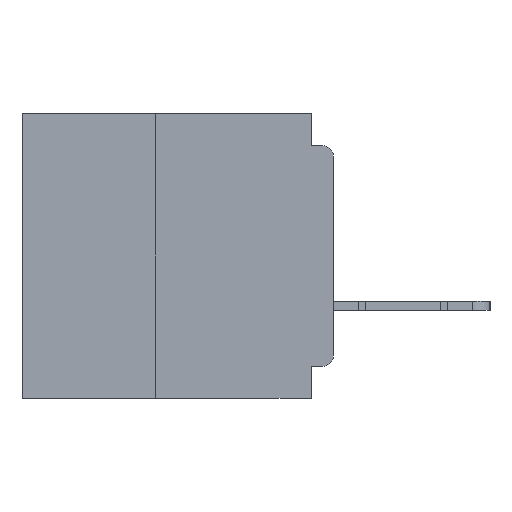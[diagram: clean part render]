
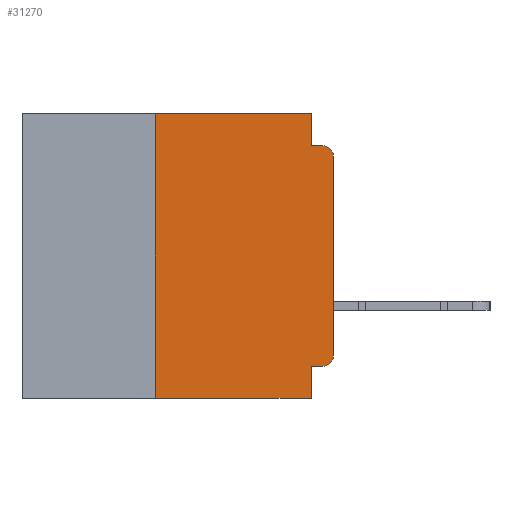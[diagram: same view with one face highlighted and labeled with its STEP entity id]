
A CAD part, left-side view. The second image highlights one B-rep face of the part: STEP entity #31270.
In plain terms, the highlighted planar face has unit normal (-1, 0, 0).
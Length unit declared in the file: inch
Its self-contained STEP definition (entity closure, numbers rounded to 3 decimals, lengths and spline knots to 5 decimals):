
#392 = EDGE_CURVE ( 'NONE', #51800, #35690, #58561, .T. ) ;
#763 = VECTOR ( 'NONE', #40756, 39.37008 ) ;
#3335 = CARTESIAN_POINT ( 'NONE',  ( 0., 0., -0.34 ) ) ;
#5136 = VERTEX_POINT ( 'NONE', #37436 ) ;
#7780 = CARTESIAN_POINT ( 'NONE',  ( 0., 0.25, -0.4 ) ) ;
#8727 = ORIENTED_EDGE ( 'NONE', *, *, #30371, .F. ) ;
#9059 = VERTEX_POINT ( 'NONE', #26474 ) ;
#10209 = DIRECTION ( 'NONE',  ( -1., 0., 0. ) ) ;
#10276 = LINE ( 'NONE', #24117, #22077 ) ;
#10562 = VECTOR ( 'NONE', #28626, 39.37008 ) ;
#10911 = LINE ( 'NONE', #58356, #49394 ) ;
#12698 = VECTOR ( 'NONE', #37609, 39.37008 ) ;
#12884 = DIRECTION ( 'NONE',  ( 0., -1., 0. ) ) ;
#13497 = VERTEX_POINT ( 'NONE', #3335 ) ;
#14047 = AXIS2_PLACEMENT_3D ( 'NONE', #47552, #17529, #52603 ) ;
#14247 = DIRECTION ( 'NONE',  ( 0., -1., 0. ) ) ;
#14360 = VERTEX_POINT ( 'NONE', #7780 ) ;
#15016 = ORIENTED_EDGE ( 'NONE', *, *, #32707, .F. ) ;
#15729 = CIRCLE ( 'NONE', #14047, 0.015 ) ;
#15766 = LINE ( 'NONE', #55743, #763 ) ;
#17529 = DIRECTION ( 'NONE',  ( -1., 0., 0. ) ) ;
#18339 = LINE ( 'NONE', #32806, #43389 ) ;
#18512 = AXIS2_PLACEMENT_3D ( 'NONE', #40192, #10209, #45269 ) ;
#19054 = AXIS2_PLACEMENT_3D ( 'NONE', #61043, #51208, #21154 ) ;
#19439 = CARTESIAN_POINT ( 'NONE',  ( 0., 0.25, 0. ) ) ;
#20060 = VECTOR ( 'NONE', #39520, 39.37008 ) ;
#20387 = EDGE_CURVE ( 'NONE', #31728, #13497, #53833, .T. ) ;
#21154 = DIRECTION ( 'NONE',  ( 0., 0., -1. ) ) ;
#21694 = VECTOR ( 'NONE', #49498, 39.37008 ) ;
#22077 = VECTOR ( 'NONE', #14247, 39.37008 ) ;
#23820 = CARTESIAN_POINT ( 'NONE',  ( 0., 0.031, -0.4 ) ) ;
#24117 = CARTESIAN_POINT ( 'NONE',  ( 0., 0.437, -0.4 ) ) ;
#26474 = CARTESIAN_POINT ( 'NONE',  ( 0., 0.015, -0.045 ) ) ;
#28338 = ORIENTED_EDGE ( 'NONE', *, *, #63743, .F. ) ;
#28626 = DIRECTION ( 'NONE',  ( 0., 0., -1. ) ) ;
#29902 = ORIENTED_EDGE ( 'NONE', *, *, #62110, .T. ) ;
#30371 = EDGE_CURVE ( 'NONE', #33110, #9059, #48378, .T. ) ;
#31270 = ADVANCED_FACE ( 'NONE', ( #56887 ), #36012, .F. ) ;
#31728 = VERTEX_POINT ( 'NONE', #34455 ) ;
#32707 = EDGE_CURVE ( 'NONE', #52388, #5136, #18339, .T. ) ;
#32806 = CARTESIAN_POINT ( 'NONE',  ( 0., 0.437, 0. ) ) ;
#33110 = VERTEX_POINT ( 'NONE', #62598 ) ;
#34455 = CARTESIAN_POINT ( 'NONE',  ( 0., 0.015, -0.355 ) ) ;
#34625 = ORIENTED_EDGE ( 'NONE', *, *, #392, .F. ) ;
#35690 = VERTEX_POINT ( 'NONE', #23820 ) ;
#36012 = PLANE ( 'NONE',  #19054 ) ;
#37436 = CARTESIAN_POINT ( 'NONE',  ( 0., 0.031, 0. ) ) ;
#37609 = DIRECTION ( 'NONE',  ( 0., 0., 1. ) ) ;
#39298 = LINE ( 'NONE', #42651, #12698 ) ;
#39520 = DIRECTION ( 'NONE',  ( 0., 0., -1. ) ) ;
#39672 = CARTESIAN_POINT ( 'NONE',  ( 0., 0.031, -0.4 ) ) ;
#40192 = CARTESIAN_POINT ( 'NONE',  ( 0., 0.015, -0.34 ) ) ;
#40756 = DIRECTION ( 'NONE',  ( 0., 1., 0. ) ) ;
#40809 = ORIENTED_EDGE ( 'NONE', *, *, #61840, .T. ) ;
#40942 = EDGE_LOOP ( 'NONE', ( #40809, #54225, #8727, #62096, #15016, #28338, #29902, #34625, #61319, #55856 ) ) ;
#42651 = CARTESIAN_POINT ( 'NONE',  ( 0., 0., 0. ) ) ;
#43389 = VECTOR ( 'NONE', #12884, 39.37008 ) ;
#45269 = DIRECTION ( 'NONE',  ( 0., 0., -1. ) ) ;
#46540 = EDGE_CURVE ( 'NONE', #53993, #9059, #15729, .T. ) ;
#47552 = CARTESIAN_POINT ( 'NONE',  ( 0., 0.015, -0.06 ) ) ;
#48378 = LINE ( 'NONE', #59573, #21694 ) ;
#48611 = CARTESIAN_POINT ( 'NONE',  ( 0., 0.031, 0. ) ) ;
#49394 = VECTOR ( 'NONE', #53537, 39.37008 ) ;
#49498 = DIRECTION ( 'NONE',  ( 0., -1., 0. ) ) ;
#49797 = CARTESIAN_POINT ( 'NONE',  ( 0., 0.031, -0.355 ) ) ;
#50616 = LINE ( 'NONE', #48611, #10562 ) ;
#51208 = DIRECTION ( 'NONE',  ( 1., 0., 0. ) ) ;
#51800 = VERTEX_POINT ( 'NONE', #49797 ) ;
#52388 = VERTEX_POINT ( 'NONE', #19439 ) ;
#52603 = DIRECTION ( 'NONE',  ( 0., 0., -1. ) ) ;
#53537 = DIRECTION ( 'NONE',  ( 0., 0., 1. ) ) ;
#53833 = CIRCLE ( 'NONE', #18512, 0.015 ) ;
#53993 = VERTEX_POINT ( 'NONE', #59917 ) ;
#54080 = EDGE_CURVE ( 'NONE', #31728, #51800, #15766, .T. ) ;
#54225 = ORIENTED_EDGE ( 'NONE', *, *, #46540, .T. ) ;
#55743 = CARTESIAN_POINT ( 'NONE',  ( 0., 0., -0.355 ) ) ;
#55856 = ORIENTED_EDGE ( 'NONE', *, *, #20387, .T. ) ;
#56887 = FACE_OUTER_BOUND ( 'NONE', #40942, .T. ) ;
#58356 = CARTESIAN_POINT ( 'NONE',  ( 0., 0.25, -0.4 ) ) ;
#58561 = LINE ( 'NONE', #39672, #20060 ) ;
#59573 = CARTESIAN_POINT ( 'NONE',  ( 0., 0., -0.045 ) ) ;
#59917 = CARTESIAN_POINT ( 'NONE',  ( 0., 0., -0.06 ) ) ;
#61043 = CARTESIAN_POINT ( 'NONE',  ( 0., 0.437, 0. ) ) ;
#61319 = ORIENTED_EDGE ( 'NONE', *, *, #54080, .F. ) ;
#61840 = EDGE_CURVE ( 'NONE', #13497, #53993, #39298, .T. ) ;
#62096 = ORIENTED_EDGE ( 'NONE', *, *, #64414, .F. ) ;
#62110 = EDGE_CURVE ( 'NONE', #14360, #35690, #10276, .T. ) ;
#62598 = CARTESIAN_POINT ( 'NONE',  ( 0., 0.031, -0.045 ) ) ;
#63743 = EDGE_CURVE ( 'NONE', #14360, #52388, #10911, .T. ) ;
#64414 = EDGE_CURVE ( 'NONE', #5136, #33110, #50616, .T. ) ;
